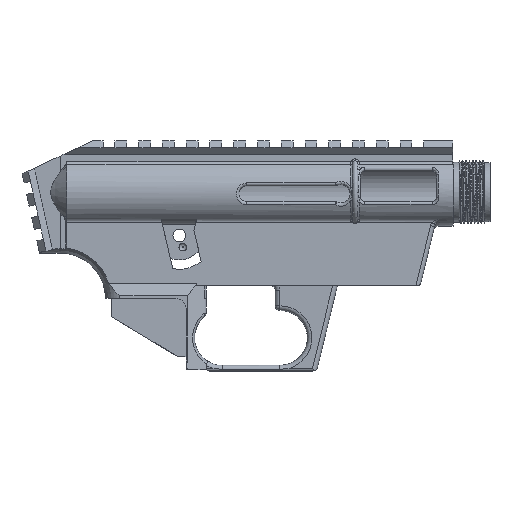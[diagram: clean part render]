
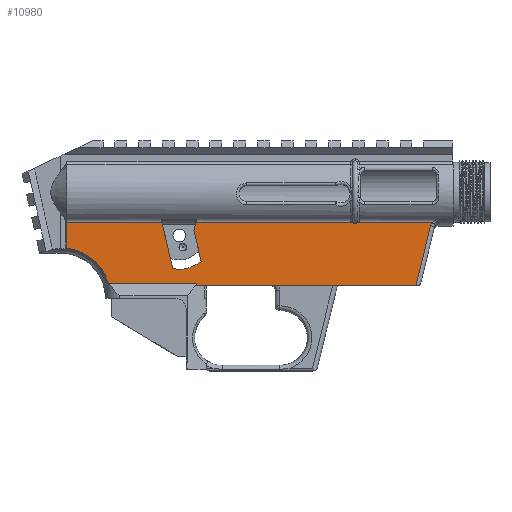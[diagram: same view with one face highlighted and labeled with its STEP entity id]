
A CAD part, left-side view. The second image highlights one B-rep face of the part: STEP entity #10980.
In plain terms, the highlighted planar face has unit normal (-1, 0, 0).
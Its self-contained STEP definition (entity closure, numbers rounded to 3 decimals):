
#329=B_SPLINE_CURVE_WITH_KNOTS('',3,(#16097,#16098,#16099,#16100,#16101,
#16102),.UNSPECIFIED.,.F.,.F.,(4,2,4),(0.,0.074,0.148),
 .UNSPECIFIED.);
#394=B_SPLINE_CURVE_WITH_KNOTS('',3,(#18947,#18948,#18949,#18950,#18951,
#18952,#18953,#18954,#18955,#18956,#18957,#18958),.UNSPECIFIED.,.F.,.F.,
(4,2,2,2,2,4),(0.,0.021,0.047,0.063,
0.077,0.097),.UNSPECIFIED.);
#395=B_SPLINE_CURVE_WITH_KNOTS('',3,(#18960,#18961,#18962,#18963,#18964,
#18965,#18966,#18967,#18968,#18969,#18970,#18971,#18972),.UNSPECIFIED.,
 .F.,.F.,(4,2,2,3,2,4),(-0.102,-0.09,-0.043,
0.,0.045,0.072),.UNSPECIFIED.);
#579=CIRCLE('',#11267,14.884);
#668=CIRCLE('',#11583,22.405);
#1236=FACE_OUTER_BOUND('',#1837,.T.);
#1837=EDGE_LOOP('',(#9318,#9319,#9320,#9321,#9322,#9323,#9324,#9325,#9326,
#9327,#9328,#9329,#9330,#9331,#9332,#9333));
#2129=LINE('',#15423,#3239);
#2135=LINE('',#15476,#3245);
#2237=LINE('',#15843,#3347);
#2280=LINE('',#16106,#3390);
#2579=LINE('',#16719,#3689);
#2633=LINE('',#16938,#3743);
#2682=LINE('',#17565,#3792);
#2683=LINE('',#17578,#3793);
#2908=LINE('',#18715,#4018);
#2920=LINE('',#18944,#4030);
#2921=LINE('',#18959,#4031);
#3239=VECTOR('',#12372,10.);
#3245=VECTOR('',#12400,10.);
#3347=VECTOR('',#12700,10.);
#3390=VECTOR('',#12839,10.);
#3689=VECTOR('',#13310,10.);
#3743=VECTOR('',#13430,10.);
#3792=VECTOR('',#13579,10.);
#3793=VECTOR('',#13586,10.);
#4018=VECTOR('',#14181,10.);
#4030=VECTOR('',#14223,10.);
#4031=VECTOR('',#14226,10.);
#4391=VERTEX_POINT('',#15421);
#4392=VERTEX_POINT('',#15422);
#4400=VERTEX_POINT('',#15474);
#4401=VERTEX_POINT('',#15475);
#4498=VERTEX_POINT('',#15837);
#4550=VERTEX_POINT('',#16094);
#4551=VERTEX_POINT('',#16096);
#4552=VERTEX_POINT('',#16105);
#4780=VERTEX_POINT('',#16717);
#4817=VERTEX_POINT('',#16933);
#4867=VERTEX_POINT('',#17562);
#4868=VERTEX_POINT('',#17564);
#4869=VERTEX_POINT('',#17577);
#5020=VERTEX_POINT('',#18710);
#5031=VERTEX_POINT('',#18793);
#5033=VERTEX_POINT('',#18946);
#5491=EDGE_CURVE('',#4391,#4392,#2129,.T.);
#5504=EDGE_CURVE('',#4400,#4401,#2135,.T.);
#5509=EDGE_CURVE('',#4392,#4400,#579,.T.);
#5654=EDGE_CURVE('',#4401,#4498,#2237,.T.);
#5727=EDGE_CURVE('',#4550,#4551,#329,.T.);
#5729=EDGE_CURVE('',#4551,#4552,#2280,.T.);
#6029=EDGE_CURVE('',#4780,#4391,#2579,.T.);
#6109=EDGE_CURVE('',#4817,#4780,#2633,.T.);
#6201=EDGE_CURVE('',#4868,#4867,#2682,.T.);
#6203=EDGE_CURVE('',#4868,#4817,#668,.T.);
#6204=EDGE_CURVE('',#4867,#4869,#2683,.T.);
#6505=EDGE_CURVE('',#5020,#4550,#2908,.T.);
#6531=EDGE_CURVE('',#4498,#5031,#2920,.T.);
#6532=EDGE_CURVE('',#5033,#5031,#394,.T.);
#6533=EDGE_CURVE('',#4552,#4869,#2921,.T.);
#6534=EDGE_CURVE('',#5020,#5033,#395,.T.);
#9318=ORIENTED_EDGE('',*,*,#6532,.T.);
#9319=ORIENTED_EDGE('',*,*,#6531,.F.);
#9320=ORIENTED_EDGE('',*,*,#5654,.F.);
#9321=ORIENTED_EDGE('',*,*,#5504,.F.);
#9322=ORIENTED_EDGE('',*,*,#5509,.F.);
#9323=ORIENTED_EDGE('',*,*,#5491,.F.);
#9324=ORIENTED_EDGE('',*,*,#6029,.F.);
#9325=ORIENTED_EDGE('',*,*,#6109,.F.);
#9326=ORIENTED_EDGE('',*,*,#6203,.F.);
#9327=ORIENTED_EDGE('',*,*,#6201,.T.);
#9328=ORIENTED_EDGE('',*,*,#6204,.T.);
#9329=ORIENTED_EDGE('',*,*,#6533,.F.);
#9330=ORIENTED_EDGE('',*,*,#5729,.F.);
#9331=ORIENTED_EDGE('',*,*,#5727,.F.);
#9332=ORIENTED_EDGE('',*,*,#6505,.F.);
#9333=ORIENTED_EDGE('',*,*,#6534,.T.);
#10469=PLANE('',#11785);
#10980=ADVANCED_FACE('',(#1236),#10469,.T.);
#11267=AXIS2_PLACEMENT_3D('',#15484,#12407,#12408);
#11583=AXIS2_PLACEMENT_3D('',#17575,#13582,#13583);
#11785=AXIS2_PLACEMENT_3D('',#18945,#14224,#14225);
#12372=DIRECTION('',(0.,-0.229,-0.973));
#12400=DIRECTION('',(0.,0.225,0.974));
#12407=DIRECTION('center_axis',(-1.,0.,0.));
#12408=DIRECTION('ref_axis',(0.,-1.,0.));
#12700=DIRECTION('',(0.,-0.225,0.974));
#12839=DIRECTION('',(0.,0.236,-0.972));
#13310=DIRECTION('',(0.,-1.,0.));
#13430=DIRECTION('',(0.,0.,1.));
#13579=DIRECTION('',(0.,-1.,0.));
#13582=DIRECTION('center_axis',(-1.,0.,0.));
#13583=DIRECTION('ref_axis',(0.,0.,1.));
#13586=DIRECTION('',(0.,0.,-1.));
#14181=DIRECTION('',(0.,-1.,0.));
#14223=DIRECTION('',(0.,-1.,0.));
#14224=DIRECTION('center_axis',(-1.,0.,0.));
#14225=DIRECTION('ref_axis',(0.,0.,1.));
#14226=DIRECTION('',(0.,1.,0.));
#15421=CARTESIAN_POINT('',(-8.42,50.391,27.845));
#15422=CARTESIAN_POINT('',(-8.42,45.62,7.575));
#15423=CARTESIAN_POINT('',(-8.42,43.577,-1.101));
#15474=CARTESIAN_POINT('',(-8.42,33.128,10.797));
#15475=CARTESIAN_POINT('',(-8.42,36.258,24.36));
#15476=CARTESIAN_POINT('',(-8.42,32.672,8.823));
#15484=CARTESIAN_POINT('Origin',(-8.42,42.724,22.175));
#15837=CARTESIAN_POINT('',(-8.42,35.445,27.888));
#15843=CARTESIAN_POINT('',(-8.42,37.307,19.808));
#16094=CARTESIAN_POINT('',(-8.42,-68.554,27.888));
#16096=CARTESIAN_POINT('',(-8.42,-67.981,26.535));
#16097=CARTESIAN_POINT('Ctrl Pts',(-8.42,-68.554,27.888));
#16098=CARTESIAN_POINT('Ctrl Pts',(-8.42,-68.423,27.68));
#16099=CARTESIAN_POINT('Ctrl Pts',(-8.42,-68.308,27.461));
#16100=CARTESIAN_POINT('Ctrl Pts',(-8.42,-68.116,27.008));
#16101=CARTESIAN_POINT('Ctrl Pts',(-8.42,-68.039,26.774));
#16102=CARTESIAN_POINT('Ctrl Pts',(-8.42,-67.981,26.535));
#16105=CARTESIAN_POINT('',(-8.42,-61.545,0.));
#16106=CARTESIAN_POINT('',(-8.42,-59.885,-6.843));
#16717=CARTESIAN_POINT('',(-8.42,92.25,27.845));
#16719=CARTESIAN_POINT('',(-8.42,0.,27.845));
#16933=CARTESIAN_POINT('',(-8.42,92.25,16.62));
#16938=CARTESIAN_POINT('',(-8.42,92.25,27.235));
#17562=CARTESIAN_POINT('',(-8.42,34.978,0.971));
#17564=CARTESIAN_POINT('',(-8.42,73.825,0.971));
#17565=CARTESIAN_POINT('',(-8.42,29.708,0.971));
#17575=CARTESIAN_POINT('Origin',(-8.42,95.25,-5.583));
#17577=CARTESIAN_POINT('',(-8.42,34.978,0.));
#17578=CARTESIAN_POINT('',(-8.42,34.978,0.));
#18710=CARTESIAN_POINT('',(-8.42,-35.664,27.888));
#18715=CARTESIAN_POINT('',(-8.42,0.,27.888));
#18793=CARTESIAN_POINT('',(-8.42,-33.329,27.888));
#18944=CARTESIAN_POINT('',(-8.42,0.,27.888));
#18945=CARTESIAN_POINT('Origin',(-8.42,0.,0.));
#18946=CARTESIAN_POINT('',(-8.42,-34.046,27.659));
#18947=CARTESIAN_POINT('Ctrl Pts',(-8.42,-34.046,27.659));
#18948=CARTESIAN_POINT('Ctrl Pts',(-8.42,-33.992,27.704));
#18949=CARTESIAN_POINT('Ctrl Pts',(-8.42,-33.933,27.741));
#18950=CARTESIAN_POINT('Ctrl Pts',(-8.42,-33.793,27.81));
#18951=CARTESIAN_POINT('Ctrl Pts',(-8.42,-33.722,27.831));
#18952=CARTESIAN_POINT('Ctrl Pts',(-8.42,-33.629,27.852));
#18953=CARTESIAN_POINT('Ctrl Pts',(-8.42,-33.594,27.859));
#18954=CARTESIAN_POINT('Ctrl Pts',(-8.42,-33.527,27.868));
#18955=CARTESIAN_POINT('Ctrl Pts',(-8.42,-33.495,27.872));
#18956=CARTESIAN_POINT('Ctrl Pts',(-8.42,-33.419,27.88));
#18957=CARTESIAN_POINT('Ctrl Pts',(-8.42,-33.377,27.884));
#18958=CARTESIAN_POINT('Ctrl Pts',(-8.42,-33.329,27.888));
#18959=CARTESIAN_POINT('',(-8.42,17.489,0.));
#18960=CARTESIAN_POINT('Ctrl Pts',(-8.42,-35.664,27.888));
#18961=CARTESIAN_POINT('Ctrl Pts',(-8.42,-35.638,27.853));
#18962=CARTESIAN_POINT('Ctrl Pts',(-8.42,-35.61,27.819));
#18963=CARTESIAN_POINT('Ctrl Pts',(-8.42,-35.478,27.674));
#18964=CARTESIAN_POINT('Ctrl Pts',(-8.42,-35.329,27.561));
#18965=CARTESIAN_POINT('Ctrl Pts',(-8.42,-35.057,27.438));
#18966=CARTESIAN_POINT('Ctrl Pts',(-8.42,-34.889,27.401));
#18967=CARTESIAN_POINT('Ctrl Pts',(-8.42,-34.746,27.401));
#18968=CARTESIAN_POINT('Ctrl Pts',(-8.42,-34.597,27.401));
#18969=CARTESIAN_POINT('Ctrl Pts',(-8.42,-34.422,27.442));
#18970=CARTESIAN_POINT('Ctrl Pts',(-8.42,-34.206,27.544));
#18971=CARTESIAN_POINT('Ctrl Pts',(-8.42,-34.122,27.597));
#18972=CARTESIAN_POINT('Ctrl Pts',(-8.42,-34.046,27.659));
